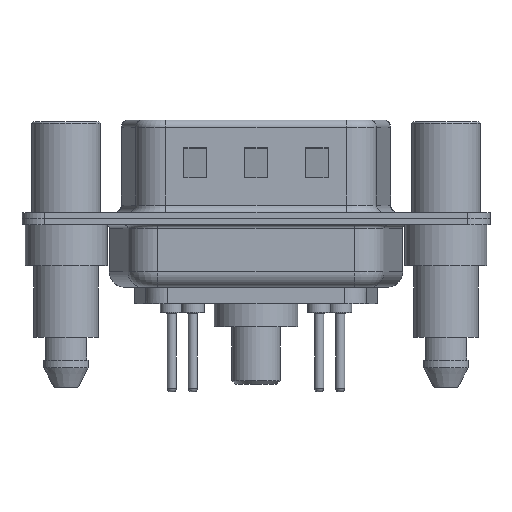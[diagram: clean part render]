
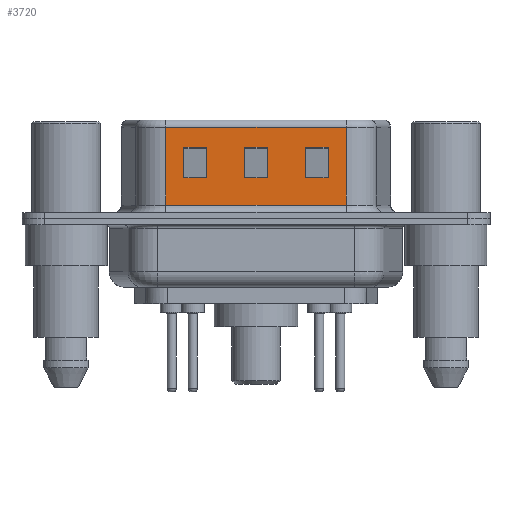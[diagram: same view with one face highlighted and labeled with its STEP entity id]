
A CAD part, front view. The second image highlights one B-rep face of the part: STEP entity #3720.
In plain terms, the highlighted planar face has unit normal (0, -1, 0).
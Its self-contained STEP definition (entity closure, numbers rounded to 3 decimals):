
#20 = CARTESIAN_POINT ( 'NONE',  ( 22.45, -4.58, 4.705 ) ) ;
#27 = ORIENTED_EDGE ( 'NONE', *, *, #11434, .T. ) ;
#105 = CARTESIAN_POINT ( 'NONE',  ( 6.55, -4.58, 6.52 ) ) ;
#198 = ORIENTED_EDGE ( 'NONE', *, *, #14148, .T. ) ;
#309 = VECTOR ( 'NONE', #15085, 1000. ) ;
#411 = VERTEX_POINT ( 'NONE', #13276 ) ;
#435 = CARTESIAN_POINT ( 'NONE',  ( 11.75, -4.58, 4.705 ) ) ;
#520 = VECTOR ( 'NONE', #17039, 1000. ) ;
#550 = LINE ( 'NONE', #13659, #7668 ) ;
#737 = EDGE_CURVE ( 'NONE', #2275, #16099, #17065, .T. ) ;
#766 = LINE ( 'NONE', #20, #309 ) ;
#773 = EDGE_LOOP ( 'NONE', ( #8154, #4709, #2739, #5771 ) ) ;
#991 = DIRECTION ( 'NONE',  ( 0., 1., 0. ) ) ;
#1169 = VECTOR ( 'NONE', #13642, 1000. ) ;
#1238 = VECTOR ( 'NONE', #15912, 1000. ) ;
#1263 = EDGE_CURVE ( 'NONE', #16099, #4934, #11917, .T. ) ;
#1434 = VECTOR ( 'NONE', #12260, 1000. ) ;
#1450 = CARTESIAN_POINT ( 'NONE',  ( 6.55, -4.58, 0.9 ) ) ;
#1793 = VERTEX_POINT ( 'NONE', #17096 ) ;
#1864 = VECTOR ( 'NONE', #15564, 1000. ) ;
#1935 = VECTOR ( 'NONE', #7540, 1000. ) ;
#2088 = EDGE_CURVE ( 'NONE', #9882, #6986, #9327, .T. ) ;
#2195 = CARTESIAN_POINT ( 'NONE',  ( 18.45, -4.58, 0.9 ) ) ;
#2275 = VERTEX_POINT ( 'NONE', #4577 ) ;
#2346 = VERTEX_POINT ( 'NONE', #16966 ) ;
#2417 = EDGE_LOOP ( 'NONE', ( #198, #27, #12324, #9366 ) ) ;
#2542 = FACE_BOUND ( 'NONE', #15270, .T. ) ;
#2688 = EDGE_CURVE ( 'NONE', #2346, #8093, #14593, .T. ) ;
#2739 = ORIENTED_EDGE ( 'NONE', *, *, #6376, .T. ) ;
#2835 = LINE ( 'NONE', #6146, #1935 ) ;
#3023 = CARTESIAN_POINT ( 'NONE',  ( 18.45, -4.58, 6.52 ) ) ;
#3034 = CARTESIAN_POINT ( 'NONE',  ( 18.45, -4.58, 6.02 ) ) ;
#3322 = VERTEX_POINT ( 'NONE', #8832 ) ;
#3420 = EDGE_CURVE ( 'NONE', #9387, #14865, #5662, .T. ) ;
#3571 = DIRECTION ( 'NONE',  ( 0., 0., -1. ) ) ;
#3695 = LINE ( 'NONE', #3023, #17510 ) ;
#3720 = ADVANCED_FACE ( 'NONE', ( #16395, #17222, #2542, #16804 ), #10503, .F. ) ;
#4176 = DIRECTION ( 'NONE',  ( -1., 0., 0. ) ) ;
#4342 = LINE ( 'NONE', #16979, #520 ) ;
#4361 = EDGE_CURVE ( 'NONE', #8093, #9838, #4926, .T. ) ;
#4551 = VECTOR ( 'NONE', #5818, 1000. ) ;
#4577 = CARTESIAN_POINT ( 'NONE',  ( 11.75, -4.58, 2.705 ) ) ;
#4709 = ORIENTED_EDGE ( 'NONE', *, *, #15425, .T. ) ;
#4719 = VECTOR ( 'NONE', #3571, 1000. ) ;
#4730 = VECTOR ( 'NONE', #7242, 1000. ) ;
#4926 = LINE ( 'NONE', #16274, #1169 ) ;
#4934 = VERTEX_POINT ( 'NONE', #5908 ) ;
#5321 = VERTEX_POINT ( 'NONE', #11649 ) ;
#5662 = LINE ( 'NONE', #6896, #1864 ) ;
#5763 = DIRECTION ( 'NONE',  ( 0., 0., 1. ) ) ;
#5771 = ORIENTED_EDGE ( 'NONE', *, *, #13752, .T. ) ;
#5818 = DIRECTION ( 'NONE',  ( 0., 0., -1. ) ) ;
#5889 = ORIENTED_EDGE ( 'NONE', *, *, #1263, .T. ) ;
#5908 = CARTESIAN_POINT ( 'NONE',  ( 13.25, -4.58, 4.705 ) ) ;
#6146 = CARTESIAN_POINT ( 'NONE',  ( 13.25, -4.58, 6.52 ) ) ;
#6376 = EDGE_CURVE ( 'NONE', #3322, #7177, #14053, .T. ) ;
#6517 = ORIENTED_EDGE ( 'NONE', *, *, #12724, .T. ) ;
#6627 = EDGE_CURVE ( 'NONE', #15284, #2275, #550, .T. ) ;
#6896 = CARTESIAN_POINT ( 'NONE',  ( 18.45, -4.58, 6.02 ) ) ;
#6984 = CARTESIAN_POINT ( 'NONE',  ( 9.25, -4.58, 4.705 ) ) ;
#6986 = VERTEX_POINT ( 'NONE', #2195 ) ;
#7177 = VERTEX_POINT ( 'NONE', #14739 ) ;
#7242 = DIRECTION ( 'NONE',  ( 0., 0., 1. ) ) ;
#7334 = ORIENTED_EDGE ( 'NONE', *, *, #6627, .T. ) ;
#7438 = ORIENTED_EDGE ( 'NONE', *, *, #3420, .T. ) ;
#7540 = DIRECTION ( 'NONE',  ( 0., 0., -1. ) ) ;
#7660 = AXIS2_PLACEMENT_3D ( 'NONE', #12291, #991, #17531 ) ;
#7668 = VECTOR ( 'NONE', #4176, 1000. ) ;
#8078 = EDGE_CURVE ( 'NONE', #14865, #9882, #15215, .T. ) ;
#8093 = VERTEX_POINT ( 'NONE', #15148 ) ;
#8154 = ORIENTED_EDGE ( 'NONE', *, *, #16282, .T. ) ;
#8832 = CARTESIAN_POINT ( 'NONE',  ( 15.75, -4.58, 2.705 ) ) ;
#8983 = CARTESIAN_POINT ( 'NONE',  ( 7.75, -4.58, 6.52 ) ) ;
#9327 = LINE ( 'NONE', #10391, #1434 ) ;
#9366 = ORIENTED_EDGE ( 'NONE', *, *, #4361, .T. ) ;
#9387 = VERTEX_POINT ( 'NONE', #3034 ) ;
#9838 = VERTEX_POINT ( 'NONE', #6984 ) ;
#9882 = VERTEX_POINT ( 'NONE', #1450 ) ;
#10199 = ORIENTED_EDGE ( 'NONE', *, *, #2088, .T. ) ;
#10391 = CARTESIAN_POINT ( 'NONE',  ( 18.45, -4.58, 0.9 ) ) ;
#10477 = EDGE_LOOP ( 'NONE', ( #12528, #7438, #12654, #10199 ) ) ;
#10503 = PLANE ( 'NONE',  #7660 ) ;
#10700 = CARTESIAN_POINT ( 'NONE',  ( 11.75, -4.58, 6.52 ) ) ;
#10917 = CARTESIAN_POINT ( 'NONE',  ( 6.55, -4.58, 6.02 ) ) ;
#11400 = CARTESIAN_POINT ( 'NONE',  ( 18.45, -4.58, 4.705 ) ) ;
#11434 = EDGE_CURVE ( 'NONE', #1793, #2346, #15732, .T. ) ;
#11649 = CARTESIAN_POINT ( 'NONE',  ( 17.25, -4.58, 2.705 ) ) ;
#11917 = LINE ( 'NONE', #11400, #1238 ) ;
#12064 = LINE ( 'NONE', #15597, #4719 ) ;
#12260 = DIRECTION ( 'NONE',  ( 1., 0., 0. ) ) ;
#12291 = CARTESIAN_POINT ( 'NONE',  ( 18.45, -4.58, 6.52 ) ) ;
#12324 = ORIENTED_EDGE ( 'NONE', *, *, #2688, .T. ) ;
#12392 = VECTOR ( 'NONE', #14791, 1000. ) ;
#12528 = ORIENTED_EDGE ( 'NONE', *, *, #13235, .F. ) ;
#12643 = ORIENTED_EDGE ( 'NONE', *, *, #737, .T. ) ;
#12654 = ORIENTED_EDGE ( 'NONE', *, *, #8078, .T. ) ;
#12724 = EDGE_CURVE ( 'NONE', #4934, #15284, #2835, .T. ) ;
#13159 = CARTESIAN_POINT ( 'NONE',  ( 22.45, -4.58, 2.705 ) ) ;
#13235 = EDGE_CURVE ( 'NONE', #9387, #6986, #3695, .T. ) ;
#13276 = CARTESIAN_POINT ( 'NONE',  ( 17.25, -4.58, 4.705 ) ) ;
#13474 = CARTESIAN_POINT ( 'NONE',  ( 14.45, -4.58, 2.705 ) ) ;
#13631 = LINE ( 'NONE', #13159, #16609 ) ;
#13642 = DIRECTION ( 'NONE',  ( 1., 0., 0. ) ) ;
#13659 = CARTESIAN_POINT ( 'NONE',  ( 18.45, -4.58, 2.705 ) ) ;
#13672 = VECTOR ( 'NONE', #17183, 1000. ) ;
#13752 = EDGE_CURVE ( 'NONE', #7177, #411, #766, .T. ) ;
#13866 = DIRECTION ( 'NONE',  ( 0., 0., -1. ) ) ;
#14053 = LINE ( 'NONE', #15044, #14452 ) ;
#14148 = EDGE_CURVE ( 'NONE', #9838, #1793, #4342, .T. ) ;
#14452 = VECTOR ( 'NONE', #5763, 1000. ) ;
#14593 = LINE ( 'NONE', #8983, #4730 ) ;
#14739 = CARTESIAN_POINT ( 'NONE',  ( 15.75, -4.58, 4.705 ) ) ;
#14791 = DIRECTION ( 'NONE',  ( -1., 0., 0. ) ) ;
#14865 = VERTEX_POINT ( 'NONE', #10917 ) ;
#15044 = CARTESIAN_POINT ( 'NONE',  ( 15.75, -4.58, 6.52 ) ) ;
#15085 = DIRECTION ( 'NONE',  ( 1., 0., 0. ) ) ;
#15148 = CARTESIAN_POINT ( 'NONE',  ( 7.75, -4.58, 4.705 ) ) ;
#15215 = LINE ( 'NONE', #105, #4551 ) ;
#15270 = EDGE_LOOP ( 'NONE', ( #5889, #6517, #7334, #12643 ) ) ;
#15284 = VERTEX_POINT ( 'NONE', #15509 ) ;
#15425 = EDGE_CURVE ( 'NONE', #5321, #3322, #13631, .T. ) ;
#15509 = CARTESIAN_POINT ( 'NONE',  ( 13.25, -4.58, 2.705 ) ) ;
#15564 = DIRECTION ( 'NONE',  ( -1., 0., 0. ) ) ;
#15597 = CARTESIAN_POINT ( 'NONE',  ( 17.25, -4.58, 6.52 ) ) ;
#15732 = LINE ( 'NONE', #13474, #12392 ) ;
#15912 = DIRECTION ( 'NONE',  ( 1., 0., 0. ) ) ;
#16099 = VERTEX_POINT ( 'NONE', #435 ) ;
#16274 = CARTESIAN_POINT ( 'NONE',  ( 14.45, -4.58, 4.705 ) ) ;
#16282 = EDGE_CURVE ( 'NONE', #411, #5321, #12064, .T. ) ;
#16395 = FACE_BOUND ( 'NONE', #2417, .T. ) ;
#16609 = VECTOR ( 'NONE', #16917, 1000. ) ;
#16804 = FACE_OUTER_BOUND ( 'NONE', #10477, .T. ) ;
#16917 = DIRECTION ( 'NONE',  ( -1., 0., 0. ) ) ;
#16966 = CARTESIAN_POINT ( 'NONE',  ( 7.75, -4.58, 2.705 ) ) ;
#16979 = CARTESIAN_POINT ( 'NONE',  ( 9.25, -4.58, 6.52 ) ) ;
#17039 = DIRECTION ( 'NONE',  ( 0., 0., -1. ) ) ;
#17065 = LINE ( 'NONE', #10700, #13672 ) ;
#17096 = CARTESIAN_POINT ( 'NONE',  ( 9.25, -4.58, 2.705 ) ) ;
#17183 = DIRECTION ( 'NONE',  ( 0., 0., 1. ) ) ;
#17222 = FACE_BOUND ( 'NONE', #773, .T. ) ;
#17510 = VECTOR ( 'NONE', #13866, 1000. ) ;
#17531 = DIRECTION ( 'NONE',  ( 0., 0., 1. ) ) ;
